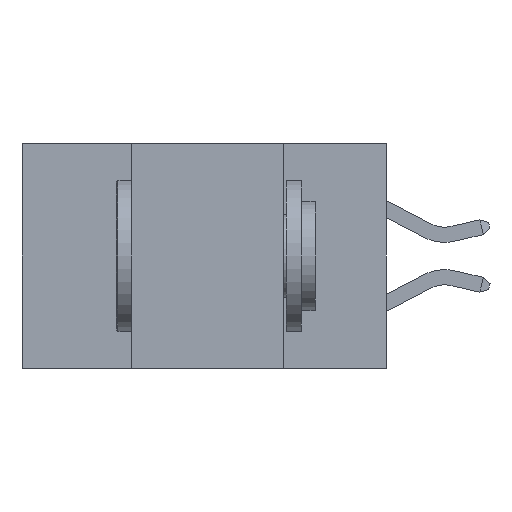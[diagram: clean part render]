
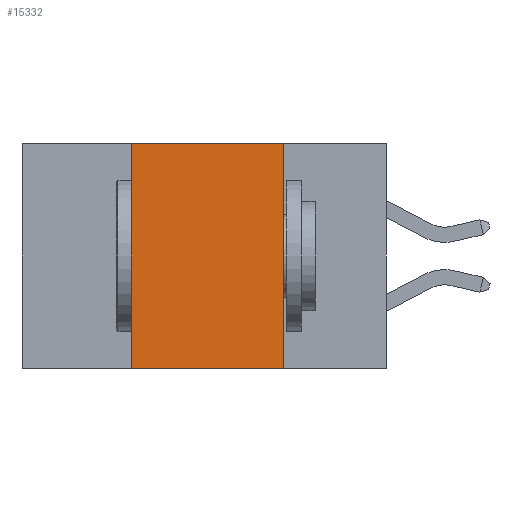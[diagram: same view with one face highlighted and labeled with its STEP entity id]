
A CAD part, left-side view. The second image highlights one B-rep face of the part: STEP entity #15332.
In plain terms, the highlighted planar face has unit normal (-1, 0, 0).
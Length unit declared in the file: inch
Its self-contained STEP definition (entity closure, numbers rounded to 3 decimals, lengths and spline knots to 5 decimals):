
#867 = LINE ( 'NONE', #17025, #7644 ) ;
#1824 = DIRECTION ( 'NONE',  ( 0., -1., 0. ) ) ;
#1825 = VERTEX_POINT ( 'NONE', #4749 ) ;
#2496 = PLANE ( 'NONE',  #6771 ) ;
#2704 = DIRECTION ( 'NONE',  ( 0., -1., 0. ) ) ;
#3766 = LINE ( 'NONE', #10500, #13544 ) ;
#3953 = EDGE_CURVE ( 'NONE', #12673, #7220, #867, .T. ) ;
#4309 = LINE ( 'NONE', #9862, #4739 ) ;
#4739 = VECTOR ( 'NONE', #1824, 39.37008 ) ;
#4749 = CARTESIAN_POINT ( 'NONE',  ( 0., 0.17, 0. ) ) ;
#4809 = CARTESIAN_POINT ( 'NONE',  ( 0., 0.17, -0.37 ) ) ;
#5800 = ORIENTED_EDGE ( 'NONE', *, *, #15668, .F. ) ;
#5873 = LINE ( 'NONE', #16469, #15942 ) ;
#6560 = DIRECTION ( 'NONE',  ( 0., 0., -1. ) ) ;
#6771 = AXIS2_PLACEMENT_3D ( 'NONE', #9186, #14466, #6560 ) ;
#6843 = EDGE_CURVE ( 'NONE', #1825, #7220, #3766, .T. ) ;
#7220 = VERTEX_POINT ( 'NONE', #4809 ) ;
#7265 = DIRECTION ( 'NONE',  ( 0., 0., 1. ) ) ;
#7644 = VECTOR ( 'NONE', #2704, 39.37008 ) ;
#9176 = VERTEX_POINT ( 'NONE', #11458 ) ;
#9186 = CARTESIAN_POINT ( 'NONE',  ( 0., 0.6, 0. ) ) ;
#9738 = FACE_OUTER_BOUND ( 'NONE', #15646, .T. ) ;
#9739 = ORIENTED_EDGE ( 'NONE', *, *, #6843, .F. ) ;
#9862 = CARTESIAN_POINT ( 'NONE',  ( 0., 0.6, 0. ) ) ;
#10310 = DIRECTION ( 'NONE',  ( 0., 0., -1. ) ) ;
#10500 = CARTESIAN_POINT ( 'NONE',  ( 0., 0.17, -0.37 ) ) ;
#11458 = CARTESIAN_POINT ( 'NONE',  ( 0., 0.42, 0. ) ) ;
#12673 = VERTEX_POINT ( 'NONE', #16987 ) ;
#13544 = VECTOR ( 'NONE', #10310, 39.37008 ) ;
#13610 = EDGE_CURVE ( 'NONE', #12673, #9176, #5873, .T. ) ;
#14466 = DIRECTION ( 'NONE',  ( 1., 0., 0. ) ) ;
#15072 = ORIENTED_EDGE ( 'NONE', *, *, #3953, .T. ) ;
#15332 = ADVANCED_FACE ( 'NONE', ( #9738 ), #2496, .F. ) ;
#15476 = ORIENTED_EDGE ( 'NONE', *, *, #13610, .F. ) ;
#15646 = EDGE_LOOP ( 'NONE', ( #9739, #5800, #15476, #15072 ) ) ;
#15668 = EDGE_CURVE ( 'NONE', #9176, #1825, #4309, .T. ) ;
#15942 = VECTOR ( 'NONE', #7265, 39.37008 ) ;
#16469 = CARTESIAN_POINT ( 'NONE',  ( 0., 0.42, -0.37 ) ) ;
#16987 = CARTESIAN_POINT ( 'NONE',  ( 0., 0.42, -0.37 ) ) ;
#17025 = CARTESIAN_POINT ( 'NONE',  ( 0., 0.6, -0.37 ) ) ;
